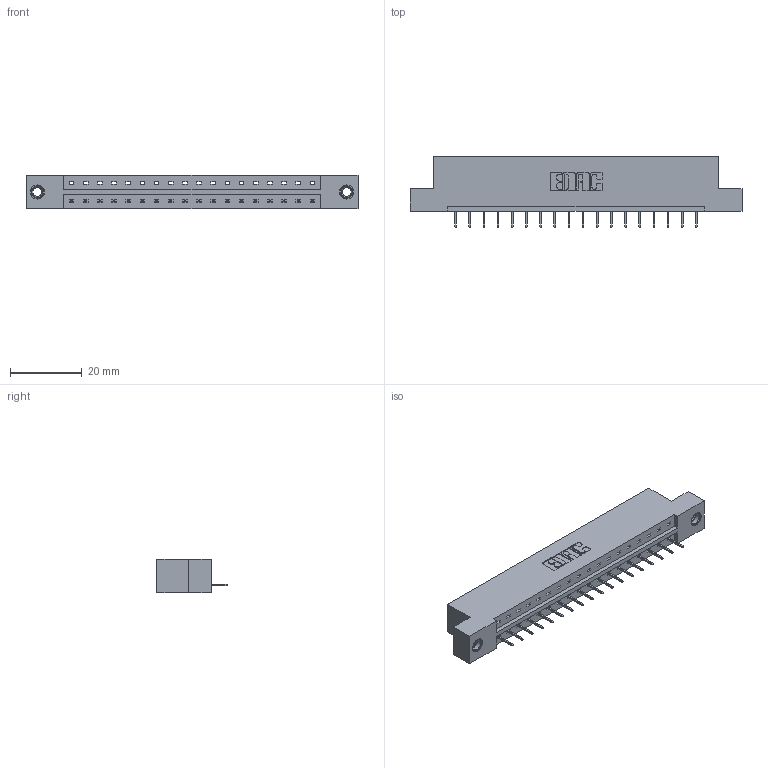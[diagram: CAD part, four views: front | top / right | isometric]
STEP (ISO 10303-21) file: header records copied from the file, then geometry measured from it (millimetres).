
FILE_DESCRIPTION (( 'STEP AP203' ), '1' );
FILE_NAME ('333-018-524-107.STEP', '2019-08-09T13:07:50', ( '' ), ( '' ), 'SwSTEP 2.0', 'SolidWorks 2016', '' );
FILE_SCHEMA (( 'CONFIG_CONTROL_DESIGN' ));
Length unit declared in the file: inch
Products named in the file (4): 333-018-524-107; 345-292-001_345-293-124; 345-250-001_345-250-005-103; 333 Part_Flush - .156 Dia - TI
Assembly tree (21 placements, depth 2):
  333-018-524-107
    333 Part_Flush - .156 Dia - TI
    345-292-001_345-293-124  x18
    345-250-001_345-250-005-103  x2
Bounding box: 92.86 x 19.69 x 9.4 mm (x, y, z)
Volume: 9053.6 mm3; surface area: 9431.9 mm2
Topology: 21 solids, 21 shells, 1290 faces, 3687 edges, 2378 vertices
Faces by surface type: plane 966, cylinder 308, cone 12, torus 4
Entity records: 15368 total; most frequent: CARTESIAN_POINT 2635, ORIENTED_EDGE 2582, DIRECTION 2305, EDGE_CURVE 1291, VECTOR 1147, LINE 1147, VERTEX_POINT 852, AXIS2_PLACEMENT_3D 579
